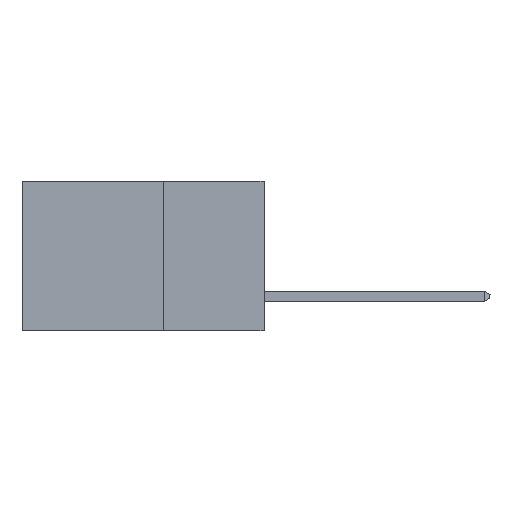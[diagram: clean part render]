
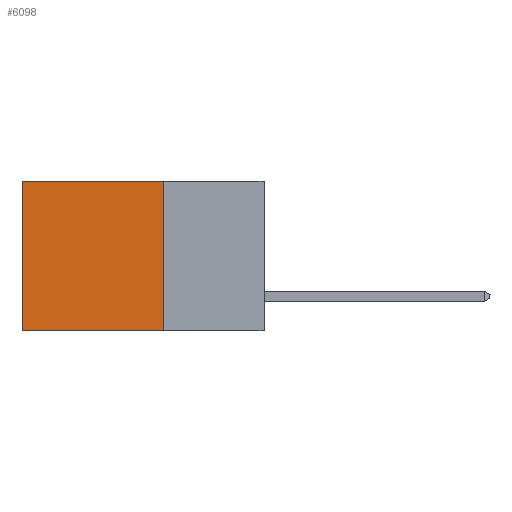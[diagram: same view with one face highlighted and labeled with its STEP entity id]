
A CAD part, left-side view. The second image highlights one B-rep face of the part: STEP entity #6098.
In plain terms, the highlighted planar face has unit normal (-1, 0, 0).
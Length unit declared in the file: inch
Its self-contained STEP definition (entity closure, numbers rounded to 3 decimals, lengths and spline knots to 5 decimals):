
#58 = EDGE_CURVE ( 'NONE', #100, #12900, #12993, .T. ) ;
#100 = VERTEX_POINT ( 'NONE', #3579 ) ;
#863 = DIRECTION ( 'NONE',  ( 0., 0., -1. ) ) ;
#2048 = DIRECTION ( 'NONE',  ( 0., 0., -1. ) ) ;
#3176 = LINE ( 'NONE', #11458, #15165 ) ;
#3299 = DIRECTION ( 'NONE',  ( 0., 0., -1. ) ) ;
#3487 = CARTESIAN_POINT ( 'NONE',  ( 0.298, 0.25, 0. ) ) ;
#3579 = CARTESIAN_POINT ( 'NONE',  ( 0.298, 0.25, 0. ) ) ;
#3628 = ORIENTED_EDGE ( 'NONE', *, *, #58, .F. ) ;
#4111 = DIRECTION ( 'NONE',  ( 0., 1., 0. ) ) ;
#4631 = CARTESIAN_POINT ( 'NONE',  ( 0.298, 0.6, 0. ) ) ;
#6046 = FACE_OUTER_BOUND ( 'NONE', #16044, .T. ) ;
#6098 = ADVANCED_FACE ( 'NONE', ( #6046 ), #10545, .F. ) ;
#6171 = VERTEX_POINT ( 'NONE', #16224 ) ;
#7276 = LINE ( 'NONE', #4631, #8136 ) ;
#7293 = LINE ( 'NONE', #13928, #14776 ) ;
#7555 = ORIENTED_EDGE ( 'NONE', *, *, #14310, .T. ) ;
#7875 = ORIENTED_EDGE ( 'NONE', *, *, #15010, .T. ) ;
#7935 = AXIS2_PLACEMENT_3D ( 'NONE', #3487, #13072, #863 ) ;
#8094 = VECTOR ( 'NONE', #2048, 39.37008 ) ;
#8136 = VECTOR ( 'NONE', #3299, 39.37008 ) ;
#8582 = CARTESIAN_POINT ( 'NONE',  ( 0.298, 0.25, -0.37 ) ) ;
#10545 = PLANE ( 'NONE',  #7935 ) ;
#11458 = CARTESIAN_POINT ( 'NONE',  ( 0.298, 0.25, -0.37 ) ) ;
#12900 = VERTEX_POINT ( 'NONE', #8582 ) ;
#12919 = CARTESIAN_POINT ( 'NONE',  ( 0.298, 0.25, 0. ) ) ;
#12993 = LINE ( 'NONE', #12919, #8094 ) ;
#13072 = DIRECTION ( 'NONE',  ( 1., 0., 0. ) ) ;
#13928 = CARTESIAN_POINT ( 'NONE',  ( 0.298, 0.25, 0. ) ) ;
#14310 = EDGE_CURVE ( 'NONE', #100, #6171, #7293, .T. ) ;
#14776 = VECTOR ( 'NONE', #4111, 39.37008 ) ;
#15010 = EDGE_CURVE ( 'NONE', #6171, #16119, #7276, .T. ) ;
#15100 = EDGE_CURVE ( 'NONE', #12900, #16119, #3176, .T. ) ;
#15165 = VECTOR ( 'NONE', #15678, 39.37008 ) ;
#15678 = DIRECTION ( 'NONE',  ( 0., 1., 0. ) ) ;
#16044 = EDGE_LOOP ( 'NONE', ( #7875, #17229, #3628, #7555 ) ) ;
#16119 = VERTEX_POINT ( 'NONE', #16479 ) ;
#16224 = CARTESIAN_POINT ( 'NONE',  ( 0.298, 0.6, 0. ) ) ;
#16479 = CARTESIAN_POINT ( 'NONE',  ( 0.298, 0.6, -0.37 ) ) ;
#17229 = ORIENTED_EDGE ( 'NONE', *, *, #15100, .F. ) ;
